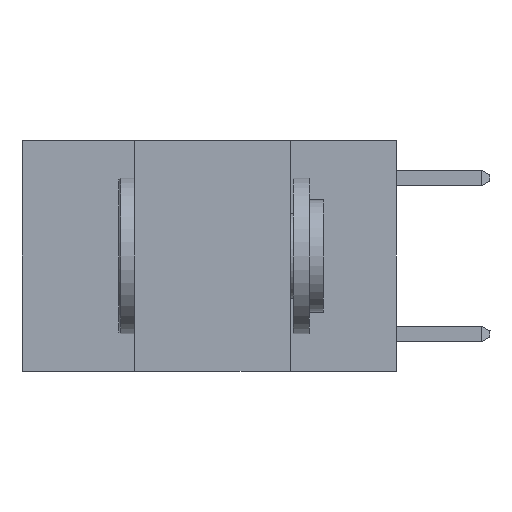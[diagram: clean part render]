
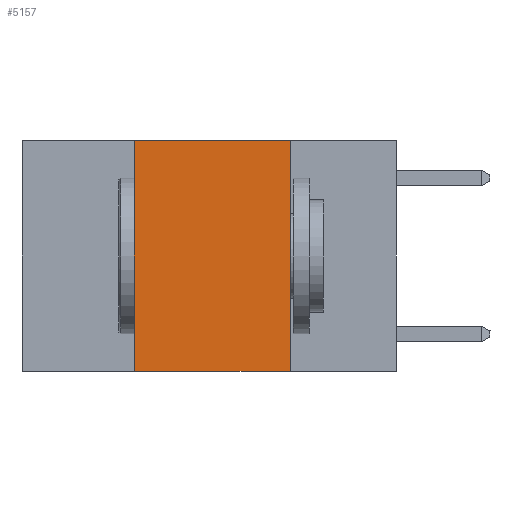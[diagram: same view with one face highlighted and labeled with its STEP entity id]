
A CAD part, left-side view. The second image highlights one B-rep face of the part: STEP entity #5157.
In plain terms, the highlighted planar face has unit normal (-1, 0, 0).
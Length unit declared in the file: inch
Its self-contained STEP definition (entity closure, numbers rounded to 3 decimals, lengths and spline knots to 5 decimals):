
#632 = LINE ( 'NONE', #8363, #8998 ) ;
#1427 = ORIENTED_EDGE ( 'NONE', *, *, #1792, .F. ) ;
#1730 = LINE ( 'NONE', #2139, #7864 ) ;
#1746 = CARTESIAN_POINT ( 'NONE',  ( 0., 0.6, -0.37 ) ) ;
#1792 = EDGE_CURVE ( 'NONE', #4396, #3089, #1730, .T. ) ;
#1944 = DIRECTION ( 'NONE',  ( 0., 0., 1. ) ) ;
#2139 = CARTESIAN_POINT ( 'NONE',  ( 0., 0.42, 0. ) ) ;
#2662 = EDGE_LOOP ( 'NONE', ( #5611, #3209, #1427, #3447 ) ) ;
#3089 = VERTEX_POINT ( 'NONE', #4513 ) ;
#3209 = ORIENTED_EDGE ( 'NONE', *, *, #6006, .F. ) ;
#3447 = ORIENTED_EDGE ( 'NONE', *, *, #10333, .T. ) ;
#3793 = CARTESIAN_POINT ( 'NONE',  ( 0., 0.42, -0.37 ) ) ;
#3850 = VECTOR ( 'NONE', #7523, 39.37008 ) ;
#4237 = VERTEX_POINT ( 'NONE', #8539 ) ;
#4396 = VERTEX_POINT ( 'NONE', #3793 ) ;
#4513 = CARTESIAN_POINT ( 'NONE',  ( 0., 0.42, 0. ) ) ;
#4719 = DIRECTION ( 'NONE',  ( 0., 0., -1. ) ) ;
#4731 = DIRECTION ( 'NONE',  ( 1., 0., 0. ) ) ;
#4754 = PLANE ( 'NONE',  #8281 ) ;
#4839 = CARTESIAN_POINT ( 'NONE',  ( 0., 0.6, 0. ) ) ;
#5050 = VECTOR ( 'NONE', #8161, 39.37008 ) ;
#5157 = ADVANCED_FACE ( 'NONE', ( #6143 ), #4754, .F. ) ;
#5611 = ORIENTED_EDGE ( 'NONE', *, *, #6447, .F. ) ;
#6006 = EDGE_CURVE ( 'NONE', #3089, #7447, #6007, .T. ) ;
#6007 = LINE ( 'NONE', #8153, #3850 ) ;
#6143 = FACE_OUTER_BOUND ( 'NONE', #2662, .T. ) ;
#6447 = EDGE_CURVE ( 'NONE', #7447, #4237, #632, .T. ) ;
#7137 = LINE ( 'NONE', #1746, #5050 ) ;
#7447 = VERTEX_POINT ( 'NONE', #9124 ) ;
#7523 = DIRECTION ( 'NONE',  ( 0., -1., 0. ) ) ;
#7864 = VECTOR ( 'NONE', #1944, 39.37008 ) ;
#8153 = CARTESIAN_POINT ( 'NONE',  ( 0., 0.6, 0. ) ) ;
#8161 = DIRECTION ( 'NONE',  ( 0., -1., 0. ) ) ;
#8281 = AXIS2_PLACEMENT_3D ( 'NONE', #4839, #4731, #4719 ) ;
#8303 = DIRECTION ( 'NONE',  ( 0., 0., -1. ) ) ;
#8363 = CARTESIAN_POINT ( 'NONE',  ( 0., 0.17, 0. ) ) ;
#8539 = CARTESIAN_POINT ( 'NONE',  ( 0., 0.17, -0.37 ) ) ;
#8998 = VECTOR ( 'NONE', #8303, 39.37008 ) ;
#9124 = CARTESIAN_POINT ( 'NONE',  ( 0., 0.17, 0. ) ) ;
#10333 = EDGE_CURVE ( 'NONE', #4396, #4237, #7137, .T. ) ;
